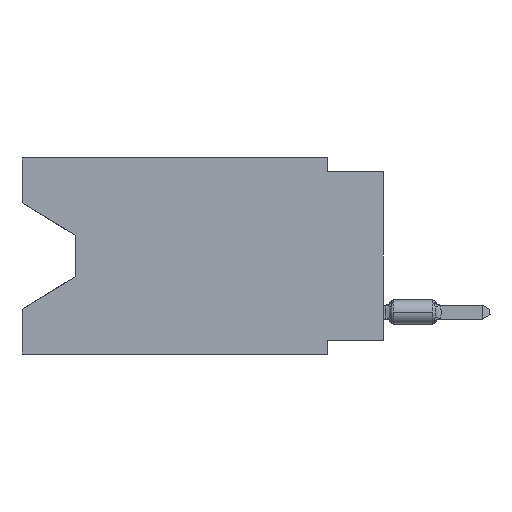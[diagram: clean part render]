
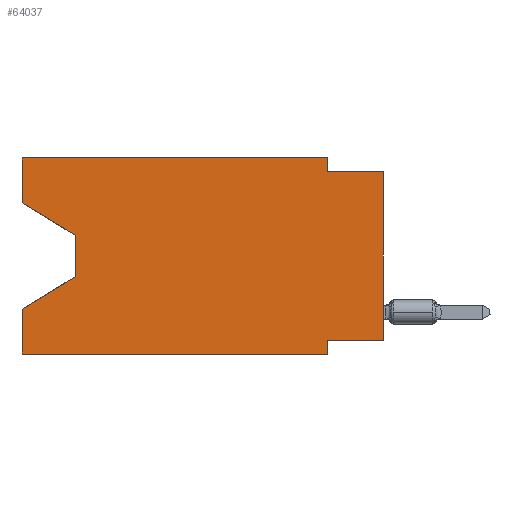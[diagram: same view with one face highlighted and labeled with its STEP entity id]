
A CAD part, left-side view. The second image highlights one B-rep face of the part: STEP entity #64037.
In plain terms, the highlighted planar face has unit normal (-1, 0, 0).
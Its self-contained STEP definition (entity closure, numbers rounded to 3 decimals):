
#404 = VECTOR ( 'NONE', #30357, 1000. ) ;
#1407 = VECTOR ( 'NONE', #84033, 1000. ) ;
#1915 = EDGE_CURVE ( 'NONE', #4485, #61800, #42607, .T. ) ;
#2230 = DIRECTION ( 'NONE',  ( 1., 0., 0. ) ) ;
#3866 = CARTESIAN_POINT ( 'NONE',  ( 0., 16.383, -8.89 ) ) ;
#4310 = EDGE_CURVE ( 'NONE', #36655, #23210, #36782, .T. ) ;
#4485 = VERTEX_POINT ( 'NONE', #64547 ) ;
#5270 = VECTOR ( 'NONE', #73868, 1000. ) ;
#7296 = CARTESIAN_POINT ( 'NONE',  ( 0., 13.97, -3.505 ) ) ;
#8134 = LINE ( 'NONE', #25676, #31007 ) ;
#8638 = CARTESIAN_POINT ( 'NONE',  ( 0., 13.97, -3.505 ) ) ;
#9136 = VERTEX_POINT ( 'NONE', #55193 ) ;
#9768 = CARTESIAN_POINT ( 'NONE',  ( 0., 16.383, -6.852 ) ) ;
#11111 = CARTESIAN_POINT ( 'NONE',  ( 0., 16.383, -2.038 ) ) ;
#11825 = ORIENTED_EDGE ( 'NONE', *, *, #21675, .T. ) ;
#12020 = ORIENTED_EDGE ( 'NONE', *, *, #62899, .F. ) ;
#12962 = VERTEX_POINT ( 'NONE', #54158 ) ;
#13021 = DIRECTION ( 'NONE',  ( 0., 0., -1. ) ) ;
#13094 = LINE ( 'NONE', #25940, #49211 ) ;
#13125 = CARTESIAN_POINT ( 'NONE',  ( 0., 2.54, -8.255 ) ) ;
#14212 = PLANE ( 'NONE',  #32643 ) ;
#14957 = VECTOR ( 'NONE', #24003, 1000. ) ;
#15897 = EDGE_CURVE ( 'NONE', #19547, #71659, #82460, .T. ) ;
#16211 = ORIENTED_EDGE ( 'NONE', *, *, #59672, .F. ) ;
#19547 = VERTEX_POINT ( 'NONE', #11111 ) ;
#19959 = VECTOR ( 'NONE', #59722, 1000. ) ;
#20141 = ORIENTED_EDGE ( 'NONE', *, *, #15897, .T. ) ;
#20616 = ORIENTED_EDGE ( 'NONE', *, *, #4310, .T. ) ;
#21041 = CARTESIAN_POINT ( 'NONE',  ( 0., 2.54, 0. ) ) ;
#21042 = LINE ( 'NONE', #8638, #52956 ) ;
#21675 = EDGE_CURVE ( 'NONE', #9136, #73957, #39016, .T. ) ;
#22762 = LINE ( 'NONE', #63768, #14957 ) ;
#23210 = VERTEX_POINT ( 'NONE', #77648 ) ;
#24003 = DIRECTION ( 'NONE',  ( 0., 0., 1. ) ) ;
#24753 = ORIENTED_EDGE ( 'NONE', *, *, #33028, .T. ) ;
#25676 = CARTESIAN_POINT ( 'NONE',  ( 0., 0., -0.635 ) ) ;
#25940 = CARTESIAN_POINT ( 'NONE',  ( 0., 0., 0. ) ) ;
#28284 = DIRECTION ( 'NONE',  ( 0., 0., -1. ) ) ;
#30357 = DIRECTION ( 'NONE',  ( 0., -1., 0. ) ) ;
#31007 = VECTOR ( 'NONE', #34212, 1000. ) ;
#31895 = LINE ( 'NONE', #46437, #1407 ) ;
#32531 = EDGE_CURVE ( 'NONE', #19547, #52970, #22762, .T. ) ;
#32643 = AXIS2_PLACEMENT_3D ( 'NONE', #48407, #2230, #79197 ) ;
#33028 = EDGE_CURVE ( 'NONE', #4485, #33158, #13094, .T. ) ;
#33158 = VERTEX_POINT ( 'NONE', #55389 ) ;
#34212 = DIRECTION ( 'NONE',  ( 0., -1., 0. ) ) ;
#34707 = LINE ( 'NONE', #21041, #69239 ) ;
#36164 = DIRECTION ( 'NONE',  ( 0., 1., 0. ) ) ;
#36655 = VERTEX_POINT ( 'NONE', #36740 ) ;
#36740 = CARTESIAN_POINT ( 'NONE',  ( 0., 16.383, -8.89 ) ) ;
#36782 = LINE ( 'NONE', #3866, #404 ) ;
#38797 = CARTESIAN_POINT ( 'NONE',  ( 0., 16.383, 0. ) ) ;
#39016 = LINE ( 'NONE', #55461, #5270 ) ;
#40599 = EDGE_CURVE ( 'NONE', #36655, #73957, #31895, .T. ) ;
#40721 = FACE_OUTER_BOUND ( 'NONE', #45593, .T. ) ;
#41876 = VECTOR ( 'NONE', #13021, 1000. ) ;
#41935 = ORIENTED_EDGE ( 'NONE', *, *, #40599, .F. ) ;
#42346 = DIRECTION ( 'NONE',  ( 0., -0.855, -0.519 ) ) ;
#42607 = LINE ( 'NONE', #62670, #46738 ) ;
#45593 = EDGE_LOOP ( 'NONE', ( #20141, #60440, #11825, #41935, #20616, #84164, #60648, #24753, #70225, #12020, #16211, #52032 ) ) ;
#46035 = DIRECTION ( 'NONE',  ( 0., 0., 1. ) ) ;
#46437 = CARTESIAN_POINT ( 'NONE',  ( 0., 16.383, 0. ) ) ;
#46684 = VERTEX_POINT ( 'NONE', #56900 ) ;
#46738 = VECTOR ( 'NONE', #36164, 1000. ) ;
#46934 = EDGE_CURVE ( 'NONE', #12962, #33158, #8134, .T. ) ;
#47126 = DIRECTION ( 'NONE',  ( 0., 0., -1. ) ) ;
#48407 = CARTESIAN_POINT ( 'NONE',  ( 0., 16.383, 0. ) ) ;
#49211 = VECTOR ( 'NONE', #46035, 1000. ) ;
#52032 = ORIENTED_EDGE ( 'NONE', *, *, #32531, .F. ) ;
#52231 = EDGE_CURVE ( 'NONE', #71659, #9136, #21042, .T. ) ;
#52956 = VECTOR ( 'NONE', #47126, 1000. ) ;
#52970 = VERTEX_POINT ( 'NONE', #78010 ) ;
#54158 = CARTESIAN_POINT ( 'NONE',  ( 0., 2.54, -0.635 ) ) ;
#55193 = CARTESIAN_POINT ( 'NONE',  ( 0., 13.97, -5.385 ) ) ;
#55389 = CARTESIAN_POINT ( 'NONE',  ( 0., 0., -0.635 ) ) ;
#55461 = CARTESIAN_POINT ( 'NONE',  ( 0., 13.97, -5.385 ) ) ;
#56900 = CARTESIAN_POINT ( 'NONE',  ( 0., 2.54, 0. ) ) ;
#58795 = CARTESIAN_POINT ( 'NONE',  ( 0., 2.54, -8.89 ) ) ;
#59672 = EDGE_CURVE ( 'NONE', #52970, #46684, #84522, .T. ) ;
#59722 = DIRECTION ( 'NONE',  ( 0., -1., 0. ) ) ;
#60215 = EDGE_CURVE ( 'NONE', #61800, #23210, #65629, .T. ) ;
#60440 = ORIENTED_EDGE ( 'NONE', *, *, #52231, .T. ) ;
#60648 = ORIENTED_EDGE ( 'NONE', *, *, #1915, .F. ) ;
#61800 = VERTEX_POINT ( 'NONE', #13125 ) ;
#62670 = CARTESIAN_POINT ( 'NONE',  ( 0., 0., -8.255 ) ) ;
#62899 = EDGE_CURVE ( 'NONE', #46684, #12962, #34707, .T. ) ;
#63768 = CARTESIAN_POINT ( 'NONE',  ( 0., 16.383, 0. ) ) ;
#64037 = ADVANCED_FACE ( 'NONE', ( #40721 ), #14212, .F. ) ;
#64547 = CARTESIAN_POINT ( 'NONE',  ( 0., 0., -8.255 ) ) ;
#65629 = LINE ( 'NONE', #58795, #41876 ) ;
#65821 = VECTOR ( 'NONE', #42346, 1000. ) ;
#69239 = VECTOR ( 'NONE', #28284, 1000. ) ;
#70225 = ORIENTED_EDGE ( 'NONE', *, *, #46934, .F. ) ;
#71659 = VERTEX_POINT ( 'NONE', #7296 ) ;
#73868 = DIRECTION ( 'NONE',  ( 0., 0.855, -0.519 ) ) ;
#73957 = VERTEX_POINT ( 'NONE', #9768 ) ;
#77648 = CARTESIAN_POINT ( 'NONE',  ( 0., 2.54, -8.89 ) ) ;
#78010 = CARTESIAN_POINT ( 'NONE',  ( 0., 16.383, 0. ) ) ;
#79197 = DIRECTION ( 'NONE',  ( 0., 0., -1. ) ) ;
#82054 = CARTESIAN_POINT ( 'NONE',  ( 0., 16.383, -2.038 ) ) ;
#82460 = LINE ( 'NONE', #82054, #65821 ) ;
#84033 = DIRECTION ( 'NONE',  ( 0., 0., 1. ) ) ;
#84164 = ORIENTED_EDGE ( 'NONE', *, *, #60215, .F. ) ;
#84522 = LINE ( 'NONE', #38797, #19959 ) ;
